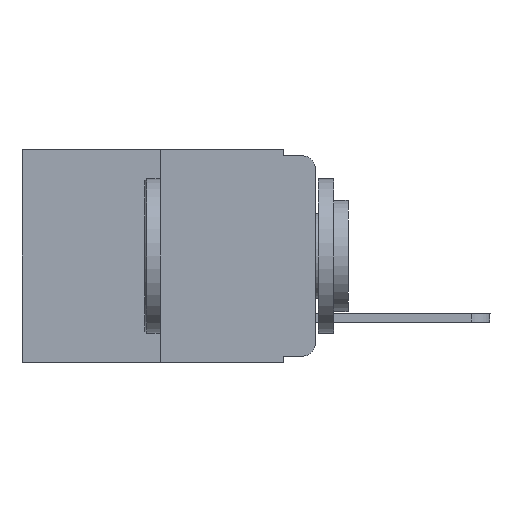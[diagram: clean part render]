
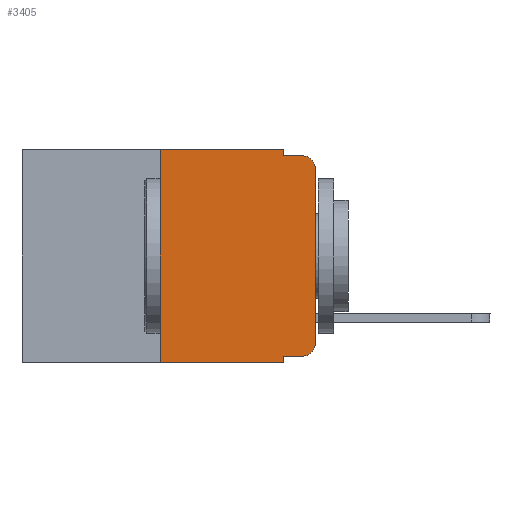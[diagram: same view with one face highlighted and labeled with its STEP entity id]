
A CAD part, left-side view. The second image highlights one B-rep face of the part: STEP entity #3405.
In plain terms, the highlighted planar face has unit normal (-1, 0, 0).
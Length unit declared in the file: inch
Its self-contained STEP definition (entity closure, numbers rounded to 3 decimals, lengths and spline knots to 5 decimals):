
#60 = LINE ( 'NONE', #19943, #4234 ) ;
#73 = ORIENTED_EDGE ( 'NONE', *, *, #507, .F. ) ;
#238 = ORIENTED_EDGE ( 'NONE', *, *, #15236, .T. ) ;
#322 = CARTESIAN_POINT ( 'NONE',  ( 0., 0.051, -0.01 ) ) ;
#507 = EDGE_CURVE ( 'NONE', #5113, #6025, #13186, .T. ) ;
#796 = CARTESIAN_POINT ( 'NONE',  ( 0., 0.25, 0. ) ) ;
#932 = LINE ( 'NONE', #17190, #2692 ) ;
#1810 = DIRECTION ( 'NONE',  ( 0., 0., -1. ) ) ;
#2090 = LINE ( 'NONE', #12612, #16370 ) ;
#2231 = CARTESIAN_POINT ( 'NONE',  ( 0., 0.02, -0.333 ) ) ;
#2312 = EDGE_CURVE ( 'NONE', #15641, #14572, #21092, .T. ) ;
#2559 = DIRECTION ( 'NONE',  ( 0., 0., 1. ) ) ;
#2692 = VECTOR ( 'NONE', #11457, 39.37008 ) ;
#2836 = CARTESIAN_POINT ( 'NONE',  ( 0., 0.02, -0.313 ) ) ;
#3079 = EDGE_CURVE ( 'NONE', #19649, #19523, #2090, .T. ) ;
#3230 = CARTESIAN_POINT ( 'NONE',  ( 0., 0.051, -0.01 ) ) ;
#3405 = ADVANCED_FACE ( 'NONE', ( #12907 ), #5562, .F. ) ;
#4234 = VECTOR ( 'NONE', #9301, 39.37008 ) ;
#4405 = CARTESIAN_POINT ( 'NONE',  ( 0., 0.473, 0. ) ) ;
#4699 = EDGE_CURVE ( 'NONE', #21260, #14572, #7476, .T. ) ;
#5113 = VERTEX_POINT ( 'NONE', #21533 ) ;
#5342 = ORIENTED_EDGE ( 'NONE', *, *, #4699, .T. ) ;
#5471 = ORIENTED_EDGE ( 'NONE', *, *, #3079, .T. ) ;
#5562 = PLANE ( 'NONE',  #20839 ) ;
#6025 = VERTEX_POINT ( 'NONE', #7016 ) ;
#7016 = CARTESIAN_POINT ( 'NONE',  ( 0., 0.25, 0. ) ) ;
#7145 = CARTESIAN_POINT ( 'NONE',  ( 0., 0.473, -0.343 ) ) ;
#7476 = CIRCLE ( 'NONE', #15663, 0.02 ) ;
#7744 = VECTOR ( 'NONE', #14087, 39.37008 ) ;
#7911 = ORIENTED_EDGE ( 'NONE', *, *, #17251, .F. ) ;
#8162 = CARTESIAN_POINT ( 'NONE',  ( 0., 0., -0.03 ) ) ;
#8205 = DIRECTION ( 'NONE',  ( -1., 0., 0. ) ) ;
#8221 = CARTESIAN_POINT ( 'NONE',  ( 0., 0.051, 0. ) ) ;
#8553 = EDGE_CURVE ( 'NONE', #19649, #19763, #932, .T. ) ;
#8596 = VECTOR ( 'NONE', #19420, 39.37008 ) ;
#8992 = DIRECTION ( 'NONE',  ( 0., -1., 0. ) ) ;
#9132 = CARTESIAN_POINT ( 'NONE',  ( 0., 0., -0.313 ) ) ;
#9188 = DIRECTION ( 'NONE',  ( -1., 0., 0. ) ) ;
#9301 = DIRECTION ( 'NONE',  ( 0., 0., 1. ) ) ;
#9411 = EDGE_CURVE ( 'NONE', #14212, #21260, #60, .T. ) ;
#9919 = ORIENTED_EDGE ( 'NONE', *, *, #19238, .F. ) ;
#10155 = CARTESIAN_POINT ( 'NONE',  ( 0., 0.02, -0.01 ) ) ;
#10505 = CARTESIAN_POINT ( 'NONE',  ( 0., 0.051, -0.333 ) ) ;
#10710 = CARTESIAN_POINT ( 'NONE',  ( 0., 0.051, 0. ) ) ;
#10851 = CARTESIAN_POINT ( 'NONE',  ( 0., 0.051, -0.343 ) ) ;
#11155 = CARTESIAN_POINT ( 'NONE',  ( 0., 0.473, 0. ) ) ;
#11169 = LINE ( 'NONE', #4405, #15012 ) ;
#11457 = DIRECTION ( 'NONE',  ( 0., 0., -1. ) ) ;
#12304 = VECTOR ( 'NONE', #2559, 39.37008 ) ;
#12571 = CARTESIAN_POINT ( 'NONE',  ( 0., 0.02, -0.03 ) ) ;
#12612 = CARTESIAN_POINT ( 'NONE',  ( 0., 0.051, -0.333 ) ) ;
#12907 = FACE_OUTER_BOUND ( 'NONE', #19996, .T. ) ;
#13186 = LINE ( 'NONE', #796, #12304 ) ;
#14087 = DIRECTION ( 'NONE',  ( 0., -1., 0. ) ) ;
#14110 = EDGE_CURVE ( 'NONE', #5113, #19763, #14153, .T. ) ;
#14153 = LINE ( 'NONE', #7145, #8596 ) ;
#14212 = VERTEX_POINT ( 'NONE', #9132 ) ;
#14242 = CIRCLE ( 'NONE', #17246, 0.02 ) ;
#14572 = VERTEX_POINT ( 'NONE', #10155 ) ;
#14691 = ORIENTED_EDGE ( 'NONE', *, *, #9411, .T. ) ;
#15012 = VECTOR ( 'NONE', #21681, 39.37008 ) ;
#15100 = DIRECTION ( 'NONE',  ( 0., 0., -1. ) ) ;
#15236 = EDGE_CURVE ( 'NONE', #19523, #14212, #14242, .T. ) ;
#15339 = DIRECTION ( 'NONE',  ( 0., 0., -1. ) ) ;
#15641 = VERTEX_POINT ( 'NONE', #322 ) ;
#15663 = AXIS2_PLACEMENT_3D ( 'NONE', #12571, #9188, #16323 ) ;
#16323 = DIRECTION ( 'NONE',  ( 0., 0., -1. ) ) ;
#16370 = VECTOR ( 'NONE', #8992, 39.37008 ) ;
#17071 = ORIENTED_EDGE ( 'NONE', *, *, #14110, .T. ) ;
#17119 = LINE ( 'NONE', #8221, #17349 ) ;
#17190 = CARTESIAN_POINT ( 'NONE',  ( 0., 0.051, 0. ) ) ;
#17246 = AXIS2_PLACEMENT_3D ( 'NONE', #2836, #8205, #15100 ) ;
#17251 = EDGE_CURVE ( 'NONE', #6025, #20197, #11169, .T. ) ;
#17349 = VECTOR ( 'NONE', #15339, 39.37008 ) ;
#17544 = ORIENTED_EDGE ( 'NONE', *, *, #2312, .F. ) ;
#17955 = DIRECTION ( 'NONE',  ( 1., 0., 0. ) ) ;
#19046 = ORIENTED_EDGE ( 'NONE', *, *, #8553, .F. ) ;
#19238 = EDGE_CURVE ( 'NONE', #20197, #15641, #17119, .T. ) ;
#19420 = DIRECTION ( 'NONE',  ( 0., -1., 0. ) ) ;
#19523 = VERTEX_POINT ( 'NONE', #2231 ) ;
#19649 = VERTEX_POINT ( 'NONE', #10505 ) ;
#19763 = VERTEX_POINT ( 'NONE', #10851 ) ;
#19943 = CARTESIAN_POINT ( 'NONE',  ( 0., 0., 0. ) ) ;
#19996 = EDGE_LOOP ( 'NONE', ( #14691, #5342, #17544, #9919, #7911, #73, #17071, #19046, #5471, #238 ) ) ;
#20197 = VERTEX_POINT ( 'NONE', #10710 ) ;
#20839 = AXIS2_PLACEMENT_3D ( 'NONE', #11155, #17955, #1810 ) ;
#21092 = LINE ( 'NONE', #3230, #7744 ) ;
#21260 = VERTEX_POINT ( 'NONE', #8162 ) ;
#21533 = CARTESIAN_POINT ( 'NONE',  ( 0., 0.25, -0.343 ) ) ;
#21681 = DIRECTION ( 'NONE',  ( 0., -1., 0. ) ) ;
